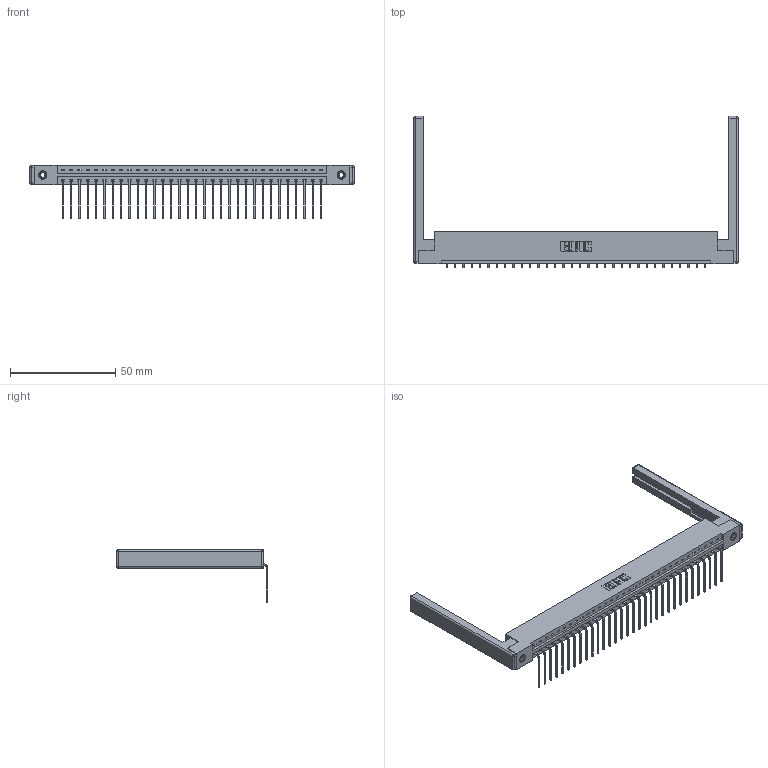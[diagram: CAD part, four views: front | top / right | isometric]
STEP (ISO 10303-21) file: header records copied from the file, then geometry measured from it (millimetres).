
FILE_DESCRIPTION (( 'STEP AP203' ), '1' );
FILE_NAME ('387-032-559-168.STEP', '2019-10-03T21:16:55', ( '' ), ( '' ), 'SwSTEP 2.0', 'SolidWorks 2016', '' );
FILE_SCHEMA (( 'CONFIG_CONTROL_DESIGN' ));
Length unit declared in the file: inch
Products named in the file (5): 307-220-068; 337 Part_Flush Mounting Lugs - 0.156 Dia-TI; 345-250-001_345-250-001-102; 387-032-559-168; 345-292-001_558 559 Tail - 1
Assembly tree (37 placements, depth 2):
  387-032-559-168
    337 Part_Flush Mounting Lugs - 0.156 Dia-TI
    345-292-001_558 559 Tail - 1  x32
    345-250-001_345-250-001-102  x2
    307-220-068  x2
Bounding box: 154.23 x 71.82 x 25.53 mm (x, y, z)
Volume: 20402.2 mm3; surface area: 21237.2 mm2
Topology: 37 solids, 37 shells, 2316 faces, 6909 edges, 4542 vertices
Faces by surface type: plane 1694, cylinder 598, cone 12, sphere 8, torus 4
Entity records: 27924 total; most frequent: CARTESIAN_POINT 4819, ORIENTED_EDGE 4776, DIRECTION 4150, EDGE_CURVE 2388, VECTOR 2210, LINE 2210, VERTEX_POINT 1582, AXIS2_PLACEMENT_3D 970
